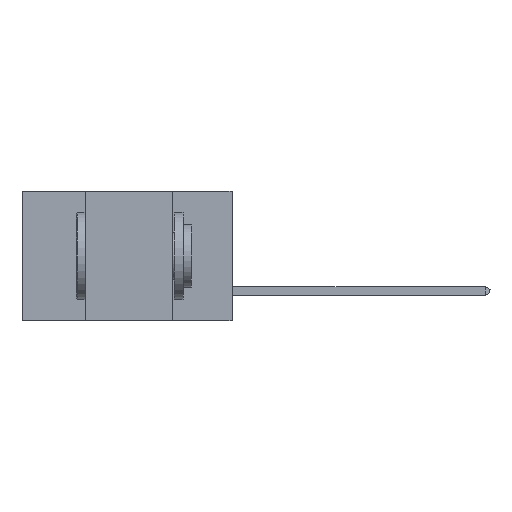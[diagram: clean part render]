
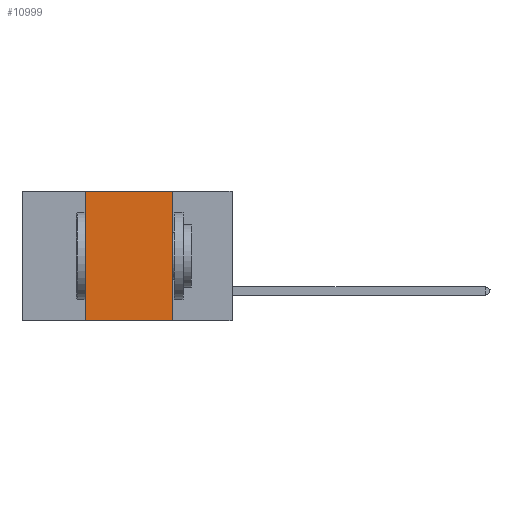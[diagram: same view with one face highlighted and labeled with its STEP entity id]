
A CAD part, left-side view. The second image highlights one B-rep face of the part: STEP entity #10999.
In plain terms, the highlighted planar face has unit normal (-1, 0, 0).
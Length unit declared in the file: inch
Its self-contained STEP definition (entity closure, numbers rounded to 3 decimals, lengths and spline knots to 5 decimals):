
#488 = EDGE_CURVE ( 'NONE', #21541, #15766, #10337, .T. ) ;
#711 = AXIS2_PLACEMENT_3D ( 'NONE', #8946, #16879, #5715 ) ;
#1547 = LINE ( 'NONE', #4090, #17552 ) ;
#2566 = VECTOR ( 'NONE', #19008, 39.37008 ) ;
#2960 = LINE ( 'NONE', #7200, #23201 ) ;
#2980 = CARTESIAN_POINT ( 'NONE',  ( 0., 0.17, -0.37 ) ) ;
#3297 = EDGE_LOOP ( 'NONE', ( #20264, #9529, #23478, #14468 ) ) ;
#4090 = CARTESIAN_POINT ( 'NONE',  ( 0., 0.17, 0. ) ) ;
#5677 = CARTESIAN_POINT ( 'NONE',  ( 0., 0.42, 0. ) ) ;
#5715 = DIRECTION ( 'NONE',  ( 0., 0., -1. ) ) ;
#6137 = DIRECTION ( 'NONE',  ( 0., 0., -1. ) ) ;
#7200 = CARTESIAN_POINT ( 'NONE',  ( 0., 0.42, 0. ) ) ;
#7272 = DIRECTION ( 'NONE',  ( 0., 0., 1. ) ) ;
#8625 = CARTESIAN_POINT ( 'NONE',  ( 0., 0.17, 0. ) ) ;
#8946 = CARTESIAN_POINT ( 'NONE',  ( 0., 0.6, 0. ) ) ;
#9529 = ORIENTED_EDGE ( 'NONE', *, *, #488, .F. ) ;
#10337 = LINE ( 'NONE', #14938, #15568 ) ;
#10988 = DIRECTION ( 'NONE',  ( 0., -1., 0. ) ) ;
#10999 = ADVANCED_FACE ( 'NONE', ( #12111 ), #18750, .F. ) ;
#11186 = EDGE_CURVE ( 'NONE', #19376, #21541, #2960, .T. ) ;
#12111 = FACE_OUTER_BOUND ( 'NONE', #3297, .T. ) ;
#12904 = EDGE_CURVE ( 'NONE', #19376, #17175, #25279, .T. ) ;
#14468 = ORIENTED_EDGE ( 'NONE', *, *, #12904, .T. ) ;
#14938 = CARTESIAN_POINT ( 'NONE',  ( 0., 0.6, 0. ) ) ;
#15568 = VECTOR ( 'NONE', #10988, 39.37008 ) ;
#15766 = VERTEX_POINT ( 'NONE', #8625 ) ;
#16879 = DIRECTION ( 'NONE',  ( 1., 0., 0. ) ) ;
#17175 = VERTEX_POINT ( 'NONE', #2980 ) ;
#17552 = VECTOR ( 'NONE', #6137, 39.37008 ) ;
#18331 = CARTESIAN_POINT ( 'NONE',  ( 0., 0.42, -0.37 ) ) ;
#18750 = PLANE ( 'NONE',  #711 ) ;
#19008 = DIRECTION ( 'NONE',  ( 0., -1., 0. ) ) ;
#19179 = CARTESIAN_POINT ( 'NONE',  ( 0., 0.6, -0.37 ) ) ;
#19376 = VERTEX_POINT ( 'NONE', #18331 ) ;
#20264 = ORIENTED_EDGE ( 'NONE', *, *, #20670, .F. ) ;
#20670 = EDGE_CURVE ( 'NONE', #15766, #17175, #1547, .T. ) ;
#21541 = VERTEX_POINT ( 'NONE', #5677 ) ;
#23201 = VECTOR ( 'NONE', #7272, 39.37008 ) ;
#23478 = ORIENTED_EDGE ( 'NONE', *, *, #11186, .F. ) ;
#25279 = LINE ( 'NONE', #19179, #2566 ) ;
